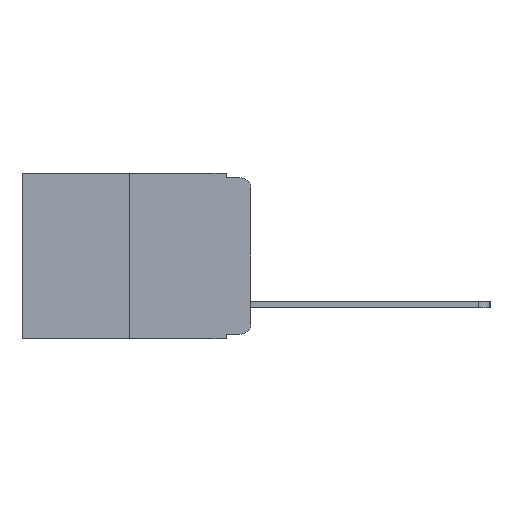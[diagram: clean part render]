
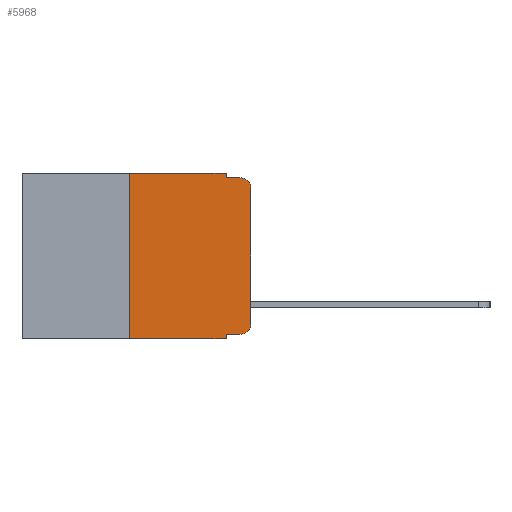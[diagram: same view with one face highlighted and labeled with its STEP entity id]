
A CAD part, left-side view. The second image highlights one B-rep face of the part: STEP entity #5968.
In plain terms, the highlighted planar face has unit normal (-1, 0, 0).
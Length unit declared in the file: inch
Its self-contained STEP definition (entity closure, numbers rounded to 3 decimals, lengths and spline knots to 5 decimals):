
#133 = AXIS2_PLACEMENT_3D ( 'NONE', #5172, #1823, #3608 ) ;
#142 = CARTESIAN_POINT ( 'NONE',  ( 0., 0.051, -0.343 ) ) ;
#170 = ORIENTED_EDGE ( 'NONE', *, *, #3084, .F. ) ;
#315 = LINE ( 'NONE', #5387, #3315 ) ;
#691 = CARTESIAN_POINT ( 'NONE',  ( 0., 0.051, 0. ) ) ;
#720 = EDGE_CURVE ( 'NONE', #1976, #10151, #8594, .T. ) ;
#803 = DIRECTION ( 'NONE',  ( 0., 0., -1. ) ) ;
#1129 = LINE ( 'NONE', #8744, #10941 ) ;
#1168 = CARTESIAN_POINT ( 'NONE',  ( 0., 0.051, -0.01 ) ) ;
#1278 = VERTEX_POINT ( 'NONE', #3627 ) ;
#1370 = VECTOR ( 'NONE', #8711, 39.37008 ) ;
#1501 = EDGE_LOOP ( 'NONE', ( #9913, #6975, #170, #2450, #8069, #5812, #2555, #7193, #8995, #7356 ) ) ;
#1618 = DIRECTION ( 'NONE',  ( 0., 0., 1. ) ) ;
#1661 = EDGE_CURVE ( 'NONE', #8957, #8424, #1129, .T. ) ;
#1823 = DIRECTION ( 'NONE',  ( -1., 0., 0. ) ) ;
#1894 = VECTOR ( 'NONE', #7324, 39.37008 ) ;
#1900 = CIRCLE ( 'NONE', #10303, 0.02 ) ;
#1968 = DIRECTION ( 'NONE',  ( 0., 0., -1. ) ) ;
#1976 = VERTEX_POINT ( 'NONE', #691 ) ;
#2385 = CARTESIAN_POINT ( 'NONE',  ( 0., 0.02, -0.313 ) ) ;
#2450 = ORIENTED_EDGE ( 'NONE', *, *, #720, .F. ) ;
#2555 = ORIENTED_EDGE ( 'NONE', *, *, #7134, .T. ) ;
#2582 = VERTEX_POINT ( 'NONE', #142 ) ;
#2615 = CIRCLE ( 'NONE', #133, 0.02 ) ;
#3084 = EDGE_CURVE ( 'NONE', #10151, #8425, #9067, .T. ) ;
#3315 = VECTOR ( 'NONE', #7144, 39.37008 ) ;
#3608 = DIRECTION ( 'NONE',  ( 0., 0., -1. ) ) ;
#3627 = CARTESIAN_POINT ( 'NONE',  ( 0., 0., -0.03 ) ) ;
#4150 = VERTEX_POINT ( 'NONE', #4963 ) ;
#4173 = VECTOR ( 'NONE', #8050, 39.37008 ) ;
#4593 = LINE ( 'NONE', #8835, #4173 ) ;
#4618 = LINE ( 'NONE', #9906, #9229 ) ;
#4730 = EDGE_CURVE ( 'NONE', #8957, #2582, #6951, .T. ) ;
#4963 = CARTESIAN_POINT ( 'NONE',  ( 0., 0.25, -0.343 ) ) ;
#4988 = EDGE_CURVE ( 'NONE', #5810, #1976, #4618, .T. ) ;
#5023 = DIRECTION ( 'NONE',  ( 1., 0., 0. ) ) ;
#5099 = CARTESIAN_POINT ( 'NONE',  ( 0., 0., -0.313 ) ) ;
#5172 = CARTESIAN_POINT ( 'NONE',  ( 0., 0.02, -0.03 ) ) ;
#5360 = CARTESIAN_POINT ( 'NONE',  ( 0., 0.051, 0. ) ) ;
#5387 = CARTESIAN_POINT ( 'NONE',  ( 0., 0.473, -0.343 ) ) ;
#5437 = VECTOR ( 'NONE', #1618, 39.37008 ) ;
#5810 = VERTEX_POINT ( 'NONE', #9154 ) ;
#5812 = ORIENTED_EDGE ( 'NONE', *, *, #9018, .F. ) ;
#5968 = ADVANCED_FACE ( 'NONE', ( #6683 ), #10081, .F. ) ;
#6097 = VECTOR ( 'NONE', #1968, 39.37008 ) ;
#6497 = CARTESIAN_POINT ( 'NONE',  ( 0., 0.051, -0.333 ) ) ;
#6618 = CARTESIAN_POINT ( 'NONE',  ( 0., 0.25, 0. ) ) ;
#6683 = FACE_OUTER_BOUND ( 'NONE', #1501, .T. ) ;
#6708 = DIRECTION ( 'NONE',  ( -1., 0., 0. ) ) ;
#6951 = LINE ( 'NONE', #5360, #6097 ) ;
#6975 = ORIENTED_EDGE ( 'NONE', *, *, #9611, .T. ) ;
#7090 = EDGE_CURVE ( 'NONE', #9991, #1278, #4593, .T. ) ;
#7134 = EDGE_CURVE ( 'NONE', #4150, #2582, #315, .T. ) ;
#7144 = DIRECTION ( 'NONE',  ( 0., -1., 0. ) ) ;
#7193 = ORIENTED_EDGE ( 'NONE', *, *, #4730, .F. ) ;
#7324 = DIRECTION ( 'NONE',  ( 0., -1., 0. ) ) ;
#7356 = ORIENTED_EDGE ( 'NONE', *, *, #9417, .T. ) ;
#7897 = DIRECTION ( 'NONE',  ( 0., -1., 0. ) ) ;
#8024 = DIRECTION ( 'NONE',  ( 0., -1., 0. ) ) ;
#8050 = DIRECTION ( 'NONE',  ( 0., 0., 1. ) ) ;
#8069 = ORIENTED_EDGE ( 'NONE', *, *, #4988, .F. ) ;
#8162 = CARTESIAN_POINT ( 'NONE',  ( 0., 0.051, -0.01 ) ) ;
#8313 = AXIS2_PLACEMENT_3D ( 'NONE', #9323, #5023, #10204 ) ;
#8424 = VERTEX_POINT ( 'NONE', #9170 ) ;
#8425 = VERTEX_POINT ( 'NONE', #10934 ) ;
#8594 = LINE ( 'NONE', #9384, #1370 ) ;
#8711 = DIRECTION ( 'NONE',  ( 0., 0., -1. ) ) ;
#8744 = CARTESIAN_POINT ( 'NONE',  ( 0., 0.051, -0.333 ) ) ;
#8835 = CARTESIAN_POINT ( 'NONE',  ( 0., 0., 0. ) ) ;
#8957 = VERTEX_POINT ( 'NONE', #6497 ) ;
#8995 = ORIENTED_EDGE ( 'NONE', *, *, #1661, .T. ) ;
#9018 = EDGE_CURVE ( 'NONE', #4150, #5810, #10960, .T. ) ;
#9067 = LINE ( 'NONE', #8162, #1894 ) ;
#9154 = CARTESIAN_POINT ( 'NONE',  ( 0., 0.25, 0. ) ) ;
#9170 = CARTESIAN_POINT ( 'NONE',  ( 0., 0.02, -0.333 ) ) ;
#9229 = VECTOR ( 'NONE', #8024, 39.37008 ) ;
#9323 = CARTESIAN_POINT ( 'NONE',  ( 0., 0.473, 0. ) ) ;
#9384 = CARTESIAN_POINT ( 'NONE',  ( 0., 0.051, 0. ) ) ;
#9417 = EDGE_CURVE ( 'NONE', #8424, #9991, #1900, .T. ) ;
#9611 = EDGE_CURVE ( 'NONE', #1278, #8425, #2615, .T. ) ;
#9906 = CARTESIAN_POINT ( 'NONE',  ( 0., 0.473, 0. ) ) ;
#9913 = ORIENTED_EDGE ( 'NONE', *, *, #7090, .T. ) ;
#9991 = VERTEX_POINT ( 'NONE', #5099 ) ;
#10081 = PLANE ( 'NONE',  #8313 ) ;
#10151 = VERTEX_POINT ( 'NONE', #1168 ) ;
#10204 = DIRECTION ( 'NONE',  ( 0., 0., -1. ) ) ;
#10303 = AXIS2_PLACEMENT_3D ( 'NONE', #2385, #6708, #803 ) ;
#10934 = CARTESIAN_POINT ( 'NONE',  ( 0., 0.02, -0.01 ) ) ;
#10941 = VECTOR ( 'NONE', #7897, 39.37008 ) ;
#10960 = LINE ( 'NONE', #6618, #5437 ) ;
